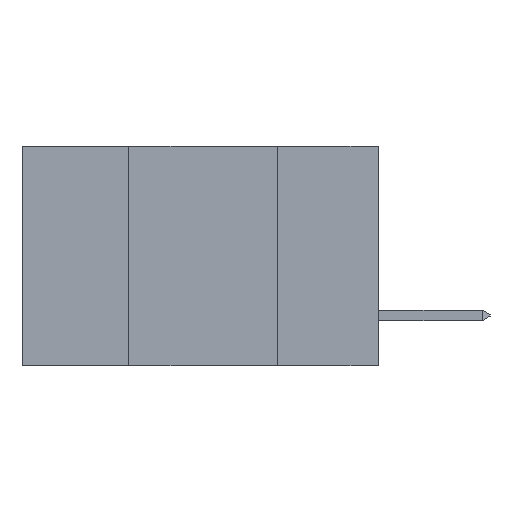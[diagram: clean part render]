
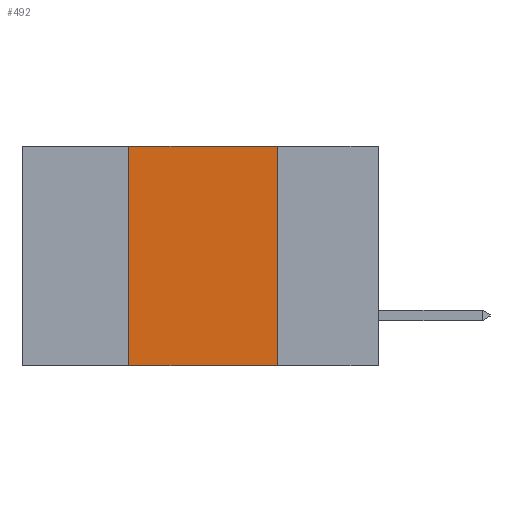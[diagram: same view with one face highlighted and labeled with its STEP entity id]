
A CAD part, left-side view. The second image highlights one B-rep face of the part: STEP entity #492.
In plain terms, the highlighted planar face has unit normal (-1, 0, 0).
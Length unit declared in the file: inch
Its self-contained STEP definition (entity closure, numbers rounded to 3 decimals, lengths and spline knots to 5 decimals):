
#492 = ADVANCED_FACE ( 'NONE', ( #23471 ), #16568, .F. ) ;
#622 = EDGE_CURVE ( 'NONE', #20939, #14131, #1841, .T. ) ;
#1841 = LINE ( 'NONE', #13093, #2421 ) ;
#2421 = VECTOR ( 'NONE', #12951, 39.37008 ) ;
#4037 = EDGE_LOOP ( 'NONE', ( #11548, #17775, #13351, #19525 ) ) ;
#4620 = CARTESIAN_POINT ( 'NONE',  ( 0., 0.42, -0.37 ) ) ;
#4816 = DIRECTION ( 'NONE',  ( 0., 0., 1. ) ) ;
#5656 = EDGE_CURVE ( 'NONE', #6219, #20939, #13076, .T. ) ;
#6219 = VERTEX_POINT ( 'NONE', #16424 ) ;
#7493 = VECTOR ( 'NONE', #13240, 39.37008 ) ;
#7587 = VERTEX_POINT ( 'NONE', #24127 ) ;
#7788 = AXIS2_PLACEMENT_3D ( 'NONE', #16387, #16360, #16274 ) ;
#8601 = VECTOR ( 'NONE', #4816, 39.37008 ) ;
#11548 = ORIENTED_EDGE ( 'NONE', *, *, #23650, .F. ) ;
#12041 = EDGE_CURVE ( 'NONE', #6219, #7587, #22435, .T. ) ;
#12951 = DIRECTION ( 'NONE',  ( 0., -1., 0. ) ) ;
#13076 = LINE ( 'NONE', #4620, #8601 ) ;
#13093 = CARTESIAN_POINT ( 'NONE',  ( 0., 0.6, 0. ) ) ;
#13240 = DIRECTION ( 'NONE',  ( 0., -1., 0. ) ) ;
#13351 = ORIENTED_EDGE ( 'NONE', *, *, #5656, .F. ) ;
#13716 = CARTESIAN_POINT ( 'NONE',  ( 0., 0.6, -0.37 ) ) ;
#14131 = VERTEX_POINT ( 'NONE', #23604 ) ;
#16274 = DIRECTION ( 'NONE',  ( 0., 0., -1. ) ) ;
#16360 = DIRECTION ( 'NONE',  ( 1., 0., 0. ) ) ;
#16387 = CARTESIAN_POINT ( 'NONE',  ( 0., 0.6, 0. ) ) ;
#16424 = CARTESIAN_POINT ( 'NONE',  ( 0., 0.42, -0.37 ) ) ;
#16568 = PLANE ( 'NONE',  #7788 ) ;
#17637 = CARTESIAN_POINT ( 'NONE',  ( 0., 0.42, 0. ) ) ;
#17775 = ORIENTED_EDGE ( 'NONE', *, *, #622, .F. ) ;
#18432 = DIRECTION ( 'NONE',  ( 0., 0., -1. ) ) ;
#18755 = LINE ( 'NONE', #21987, #22990 ) ;
#19525 = ORIENTED_EDGE ( 'NONE', *, *, #12041, .T. ) ;
#20939 = VERTEX_POINT ( 'NONE', #17637 ) ;
#21987 = CARTESIAN_POINT ( 'NONE',  ( 0., 0.17, -0.37 ) ) ;
#22435 = LINE ( 'NONE', #13716, #7493 ) ;
#22990 = VECTOR ( 'NONE', #18432, 39.37008 ) ;
#23471 = FACE_OUTER_BOUND ( 'NONE', #4037, .T. ) ;
#23604 = CARTESIAN_POINT ( 'NONE',  ( 0., 0.17, 0. ) ) ;
#23650 = EDGE_CURVE ( 'NONE', #14131, #7587, #18755, .T. ) ;
#24127 = CARTESIAN_POINT ( 'NONE',  ( 0., 0.17, -0.37 ) ) ;
